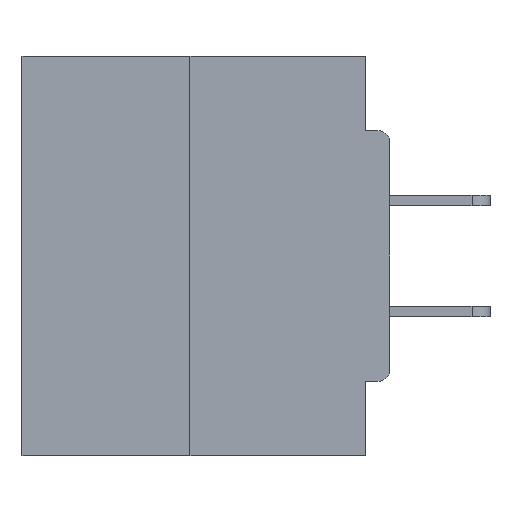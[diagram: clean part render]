
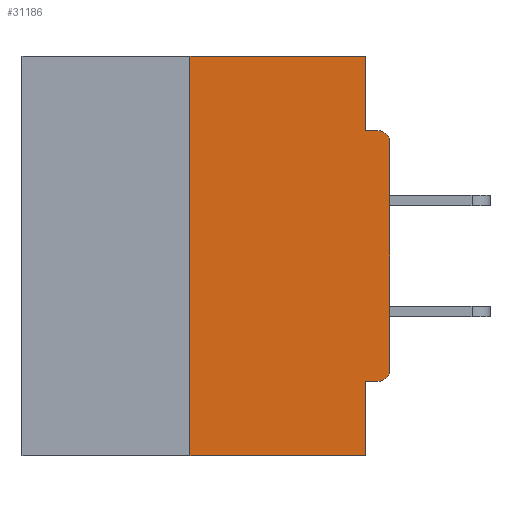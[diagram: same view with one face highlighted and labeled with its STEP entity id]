
A CAD part, left-side view. The second image highlights one B-rep face of the part: STEP entity #31186.
In plain terms, the highlighted planar face has unit normal (-1, 0, 0).
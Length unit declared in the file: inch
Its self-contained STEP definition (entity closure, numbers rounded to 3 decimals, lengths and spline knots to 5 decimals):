
#106 = CARTESIAN_POINT ( 'NONE',  ( 0., 0.25, 0. ) ) ;
#525 = EDGE_CURVE ( 'NONE', #29645, #6782, #33385, .T. ) ;
#790 = EDGE_CURVE ( 'NONE', #10418, #7125, #5428, .T. ) ;
#1502 = EDGE_LOOP ( 'NONE', ( #23621, #12430, #19453, #34608, #26391, #16460, #30710, #21352, #10768, #12394 ) ) ;
#3003 = LINE ( 'NONE', #18591, #9291 ) ;
#3077 = DIRECTION ( 'NONE',  ( 0., 0., 1. ) ) ;
#3127 = CARTESIAN_POINT ( 'NONE',  ( 0., 0.031, -0.5 ) ) ;
#4607 = DIRECTION ( 'NONE',  ( -1., 0., 0. ) ) ;
#5339 = DIRECTION ( 'NONE',  ( 0., -1., 0. ) ) ;
#5428 = LINE ( 'NONE', #15074, #18095 ) ;
#6125 = CARTESIAN_POINT ( 'NONE',  ( 0., 0.25, -0.5 ) ) ;
#6203 = EDGE_CURVE ( 'NONE', #16938, #10418, #34740, .T. ) ;
#6782 = VERTEX_POINT ( 'NONE', #11981 ) ;
#7125 = VERTEX_POINT ( 'NONE', #24598 ) ;
#7790 = VERTEX_POINT ( 'NONE', #25650 ) ;
#7883 = EDGE_CURVE ( 'NONE', #25639, #32792, #30407, .T. ) ;
#8037 = AXIS2_PLACEMENT_3D ( 'NONE', #34153, #4607, #34269 ) ;
#8267 = LINE ( 'NONE', #106, #16714 ) ;
#9291 = VECTOR ( 'NONE', #21324, 39.37008 ) ;
#10399 = DIRECTION ( 'NONE',  ( 0., 1., 0. ) ) ;
#10418 = VERTEX_POINT ( 'NONE', #32984 ) ;
#10768 = ORIENTED_EDGE ( 'NONE', *, *, #11190, .F. ) ;
#10986 = EDGE_CURVE ( 'NONE', #13962, #29645, #13937, .T. ) ;
#11190 = EDGE_CURVE ( 'NONE', #7125, #17659, #3003, .T. ) ;
#11981 = CARTESIAN_POINT ( 'NONE',  ( 0., 0., -0.1085 ) ) ;
#12394 = ORIENTED_EDGE ( 'NONE', *, *, #790, .F. ) ;
#12430 = ORIENTED_EDGE ( 'NONE', *, *, #13708, .F. ) ;
#13427 = VECTOR ( 'NONE', #5339, 39.37008 ) ;
#13708 = EDGE_CURVE ( 'NONE', #25639, #16938, #8267, .T. ) ;
#13830 = DIRECTION ( 'NONE',  ( 0., 0., -1. ) ) ;
#13937 = CIRCLE ( 'NONE', #31946, 0.015 ) ;
#13962 = VERTEX_POINT ( 'NONE', #17167 ) ;
#14088 = EDGE_CURVE ( 'NONE', #13962, #7790, #28101, .T. ) ;
#14701 = VECTOR ( 'NONE', #3077, 39.37008 ) ;
#14838 = EDGE_CURVE ( 'NONE', #6782, #17659, #27606, .T. ) ;
#15074 = CARTESIAN_POINT ( 'NONE',  ( 0., 0.031, 0. ) ) ;
#15934 = DIRECTION ( 'NONE',  ( 0., 0., -1. ) ) ;
#16460 = ORIENTED_EDGE ( 'NONE', *, *, #10986, .T. ) ;
#16472 = DIRECTION ( 'NONE',  ( 0., 0., 1. ) ) ;
#16714 = VECTOR ( 'NONE', #16472, 39.37008 ) ;
#16938 = VERTEX_POINT ( 'NONE', #18010 ) ;
#17167 = CARTESIAN_POINT ( 'NONE',  ( 0., 0.015, -0.4065 ) ) ;
#17371 = VECTOR ( 'NONE', #18592, 39.37008 ) ;
#17659 = VERTEX_POINT ( 'NONE', #30296 ) ;
#18010 = CARTESIAN_POINT ( 'NONE',  ( 0., 0.25, 0. ) ) ;
#18095 = VECTOR ( 'NONE', #23132, 39.37008 ) ;
#18337 = CARTESIAN_POINT ( 'NONE',  ( 0., 0., -0.4065 ) ) ;
#18591 = CARTESIAN_POINT ( 'NONE',  ( 0., 0., -0.0935 ) ) ;
#18592 = DIRECTION ( 'NONE',  ( 0., -1., 0. ) ) ;
#18668 = DIRECTION ( 'NONE',  ( 1., 0., 0. ) ) ;
#19453 = ORIENTED_EDGE ( 'NONE', *, *, #7883, .T. ) ;
#21278 = PLANE ( 'NONE',  #26536 ) ;
#21324 = DIRECTION ( 'NONE',  ( 0., -1., 0. ) ) ;
#21352 = ORIENTED_EDGE ( 'NONE', *, *, #14838, .T. ) ;
#21457 = VECTOR ( 'NONE', #13830, 39.37008 ) ;
#22583 = CARTESIAN_POINT ( 'NONE',  ( 0., 0.015, -0.3915 ) ) ;
#23132 = DIRECTION ( 'NONE',  ( 0., 0., -1. ) ) ;
#23441 = FACE_OUTER_BOUND ( 'NONE', #1502, .T. ) ;
#23621 = ORIENTED_EDGE ( 'NONE', *, *, #6203, .F. ) ;
#24598 = CARTESIAN_POINT ( 'NONE',  ( 0., 0.031, -0.0935 ) ) ;
#25639 = VERTEX_POINT ( 'NONE', #6125 ) ;
#25650 = CARTESIAN_POINT ( 'NONE',  ( 0., 0.031, -0.4065 ) ) ;
#26391 = ORIENTED_EDGE ( 'NONE', *, *, #14088, .F. ) ;
#26535 = LINE ( 'NONE', #3127, #21457 ) ;
#26536 = AXIS2_PLACEMENT_3D ( 'NONE', #34897, #18668, #15934 ) ;
#26824 = CARTESIAN_POINT ( 'NONE',  ( 0., 0.46, -0.5 ) ) ;
#27142 = CARTESIAN_POINT ( 'NONE',  ( 0., 0.031, -0.5 ) ) ;
#27606 = CIRCLE ( 'NONE', #8037, 0.015 ) ;
#28101 = LINE ( 'NONE', #18337, #32387 ) ;
#29053 = EDGE_CURVE ( 'NONE', #7790, #32792, #26535, .T. ) ;
#29074 = CARTESIAN_POINT ( 'NONE',  ( 0., 0., -0.3915 ) ) ;
#29355 = CARTESIAN_POINT ( 'NONE',  ( 0., 0.46, 0. ) ) ;
#29645 = VERTEX_POINT ( 'NONE', #29074 ) ;
#30010 = CARTESIAN_POINT ( 'NONE',  ( 0., 0., 0. ) ) ;
#30296 = CARTESIAN_POINT ( 'NONE',  ( 0., 0.015, -0.0935 ) ) ;
#30407 = LINE ( 'NONE', #26824, #13427 ) ;
#30710 = ORIENTED_EDGE ( 'NONE', *, *, #525, .T. ) ;
#31186 = ADVANCED_FACE ( 'NONE', ( #23441 ), #21278, .F. ) ;
#31234 = DIRECTION ( 'NONE',  ( -1., 0., 0. ) ) ;
#31946 = AXIS2_PLACEMENT_3D ( 'NONE', #22583, #31234, #33704 ) ;
#32387 = VECTOR ( 'NONE', #10399, 39.37008 ) ;
#32792 = VERTEX_POINT ( 'NONE', #27142 ) ;
#32984 = CARTESIAN_POINT ( 'NONE',  ( 0., 0.031, 0. ) ) ;
#33385 = LINE ( 'NONE', #30010, #14701 ) ;
#33704 = DIRECTION ( 'NONE',  ( 0., 0., -1. ) ) ;
#34153 = CARTESIAN_POINT ( 'NONE',  ( 0., 0.015, -0.1085 ) ) ;
#34269 = DIRECTION ( 'NONE',  ( 0., 0., -1. ) ) ;
#34608 = ORIENTED_EDGE ( 'NONE', *, *, #29053, .F. ) ;
#34740 = LINE ( 'NONE', #29355, #17371 ) ;
#34897 = CARTESIAN_POINT ( 'NONE',  ( 0., 0.46, 0. ) ) ;
